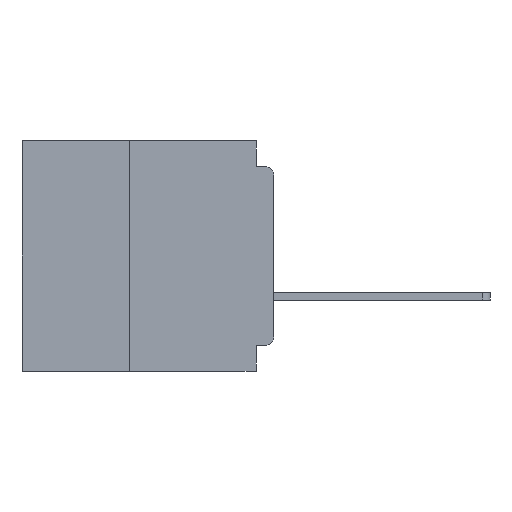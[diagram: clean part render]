
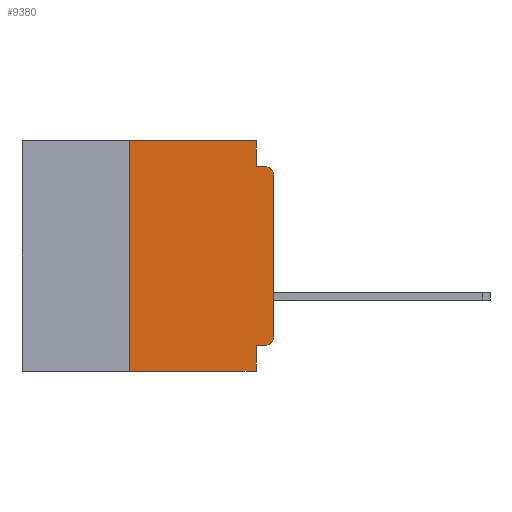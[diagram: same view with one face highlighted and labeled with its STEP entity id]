
A CAD part, left-side view. The second image highlights one B-rep face of the part: STEP entity #9380.
In plain terms, the highlighted planar face has unit normal (-1, 0, 0).
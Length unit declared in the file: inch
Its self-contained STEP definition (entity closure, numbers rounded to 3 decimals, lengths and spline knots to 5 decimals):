
#149 = VECTOR ( 'NONE', #37986, 39.37008 ) ;
#240 = CARTESIAN_POINT ( 'NONE',  ( 0., 0.25, -0.4 ) ) ;
#1936 = CARTESIAN_POINT ( 'NONE',  ( 0., 0.031, -0.4 ) ) ;
#2148 = CARTESIAN_POINT ( 'NONE',  ( 0., 0., -0.06 ) ) ;
#2951 = CARTESIAN_POINT ( 'NONE',  ( 0., 0.031, 0. ) ) ;
#3127 = DIRECTION ( 'NONE',  ( 0., 0., 1. ) ) ;
#3600 = DIRECTION ( 'NONE',  ( -1., 0., 0. ) ) ;
#4608 = CARTESIAN_POINT ( 'NONE',  ( 0., 0.015, -0.355 ) ) ;
#8284 = VERTEX_POINT ( 'NONE', #65290 ) ;
#9380 = ADVANCED_FACE ( 'NONE', ( #51940 ), #59889, .F. ) ;
#9666 = LINE ( 'NONE', #52391, #60718 ) ;
#10166 = CARTESIAN_POINT ( 'NONE',  ( 0., 0.031, -0.4 ) ) ;
#10296 = ORIENTED_EDGE ( 'NONE', *, *, #21669, .T. ) ;
#11012 = VERTEX_POINT ( 'NONE', #2148 ) ;
#12674 = EDGE_CURVE ( 'NONE', #8284, #19812, #53172, .T. ) ;
#12749 = DIRECTION ( 'NONE',  ( 0., -1., 0. ) ) ;
#13297 = DIRECTION ( 'NONE',  ( 0., 0., 1. ) ) ;
#14009 = CARTESIAN_POINT ( 'NONE',  ( 0., 0.015, -0.045 ) ) ;
#14121 = ORIENTED_EDGE ( 'NONE', *, *, #12674, .F. ) ;
#17058 = VERTEX_POINT ( 'NONE', #19544 ) ;
#17095 = ORIENTED_EDGE ( 'NONE', *, *, #65414, .F. ) ;
#18758 = VERTEX_POINT ( 'NONE', #32168 ) ;
#19027 = CIRCLE ( 'NONE', #44852, 0.015 ) ;
#19283 = CARTESIAN_POINT ( 'NONE',  ( 0., 0.437, 0. ) ) ;
#19544 = CARTESIAN_POINT ( 'NONE',  ( 0., 0.031, -0.045 ) ) ;
#19812 = VERTEX_POINT ( 'NONE', #10166 ) ;
#20603 = VERTEX_POINT ( 'NONE', #42992 ) ;
#20674 = VECTOR ( 'NONE', #65922, 39.37008 ) ;
#20716 = CARTESIAN_POINT ( 'NONE',  ( 0., 0.015, -0.06 ) ) ;
#21669 = EDGE_CURVE ( 'NONE', #22432, #18758, #19027, .T. ) ;
#22432 = VERTEX_POINT ( 'NONE', #4608 ) ;
#23365 = VERTEX_POINT ( 'NONE', #2951 ) ;
#24122 = AXIS2_PLACEMENT_3D ( 'NONE', #19283, #29618, #64959 ) ;
#25891 = DIRECTION ( 'NONE',  ( 0., 0., -1. ) ) ;
#27296 = VERTEX_POINT ( 'NONE', #14009 ) ;
#27741 = LINE ( 'NONE', #39126, #53076 ) ;
#29443 = DIRECTION ( 'NONE',  ( 0., 1., 0. ) ) ;
#29618 = DIRECTION ( 'NONE',  ( 1., 0., 0. ) ) ;
#29685 = LINE ( 'NONE', #36740, #41534 ) ;
#29822 = ORIENTED_EDGE ( 'NONE', *, *, #62243, .F. ) ;
#30301 = AXIS2_PLACEMENT_3D ( 'NONE', #20716, #56223, #25891 ) ;
#30585 = CARTESIAN_POINT ( 'NONE',  ( 0., 0.031, 0. ) ) ;
#32168 = CARTESIAN_POINT ( 'NONE',  ( 0., 0., -0.34 ) ) ;
#33910 = EDGE_CURVE ( 'NONE', #52110, #19812, #9666, .T. ) ;
#34001 = ORIENTED_EDGE ( 'NONE', *, *, #48146, .F. ) ;
#34531 = CARTESIAN_POINT ( 'NONE',  ( 0., 0.015, -0.34 ) ) ;
#36740 = CARTESIAN_POINT ( 'NONE',  ( 0., 0.437, 0. ) ) ;
#37098 = DIRECTION ( 'NONE',  ( 0., -1., 0. ) ) ;
#37172 = CIRCLE ( 'NONE', #30301, 0.015 ) ;
#37606 = ORIENTED_EDGE ( 'NONE', *, *, #45199, .T. ) ;
#37708 = VECTOR ( 'NONE', #13297, 39.37008 ) ;
#37986 = DIRECTION ( 'NONE',  ( 0., 0., -1. ) ) ;
#39126 = CARTESIAN_POINT ( 'NONE',  ( 0., 0.25, -0.4 ) ) ;
#39611 = DIRECTION ( 'NONE',  ( 0., 0., -1. ) ) ;
#40992 = EDGE_CURVE ( 'NONE', #22432, #8284, #56895, .T. ) ;
#41534 = VECTOR ( 'NONE', #61947, 39.37008 ) ;
#41649 = ORIENTED_EDGE ( 'NONE', *, *, #52597, .F. ) ;
#42941 = LINE ( 'NONE', #30585, #20674 ) ;
#42992 = CARTESIAN_POINT ( 'NONE',  ( 0., 0.25, 0. ) ) ;
#43366 = CARTESIAN_POINT ( 'NONE',  ( 0., 0., -0.045 ) ) ;
#43459 = VECTOR ( 'NONE', #29443, 39.37008 ) ;
#44577 = ORIENTED_EDGE ( 'NONE', *, *, #65050, .T. ) ;
#44852 = AXIS2_PLACEMENT_3D ( 'NONE', #34531, #3600, #39611 ) ;
#45199 = EDGE_CURVE ( 'NONE', #18758, #11012, #51175, .T. ) ;
#48146 = EDGE_CURVE ( 'NONE', #17058, #27296, #63476, .T. ) ;
#49545 = CARTESIAN_POINT ( 'NONE',  ( 0., 0., -0.355 ) ) ;
#51175 = LINE ( 'NONE', #63999, #37708 ) ;
#51940 = FACE_OUTER_BOUND ( 'NONE', #61736, .T. ) ;
#52110 = VERTEX_POINT ( 'NONE', #240 ) ;
#52391 = CARTESIAN_POINT ( 'NONE',  ( 0., 0.437, -0.4 ) ) ;
#52597 = EDGE_CURVE ( 'NONE', #23365, #17058, #42941, .T. ) ;
#53076 = VECTOR ( 'NONE', #3127, 39.37008 ) ;
#53172 = LINE ( 'NONE', #1936, #149 ) ;
#56223 = DIRECTION ( 'NONE',  ( -1., 0., 0. ) ) ;
#56895 = LINE ( 'NONE', #49545, #43459 ) ;
#58113 = ORIENTED_EDGE ( 'NONE', *, *, #40992, .F. ) ;
#59889 = PLANE ( 'NONE',  #24122 ) ;
#60088 = ORIENTED_EDGE ( 'NONE', *, *, #33910, .T. ) ;
#60718 = VECTOR ( 'NONE', #37098, 39.37008 ) ;
#61736 = EDGE_LOOP ( 'NONE', ( #37606, #44577, #34001, #41649, #29822, #17095, #60088, #14121, #58113, #10296 ) ) ;
#61947 = DIRECTION ( 'NONE',  ( 0., -1., 0. ) ) ;
#62243 = EDGE_CURVE ( 'NONE', #20603, #23365, #29685, .T. ) ;
#63476 = LINE ( 'NONE', #43366, #64151 ) ;
#63999 = CARTESIAN_POINT ( 'NONE',  ( 0., 0., 0. ) ) ;
#64151 = VECTOR ( 'NONE', #12749, 39.37008 ) ;
#64959 = DIRECTION ( 'NONE',  ( 0., 0., -1. ) ) ;
#65050 = EDGE_CURVE ( 'NONE', #11012, #27296, #37172, .T. ) ;
#65290 = CARTESIAN_POINT ( 'NONE',  ( 0., 0.031, -0.355 ) ) ;
#65414 = EDGE_CURVE ( 'NONE', #52110, #20603, #27741, .T. ) ;
#65922 = DIRECTION ( 'NONE',  ( 0., 0., -1. ) ) ;
